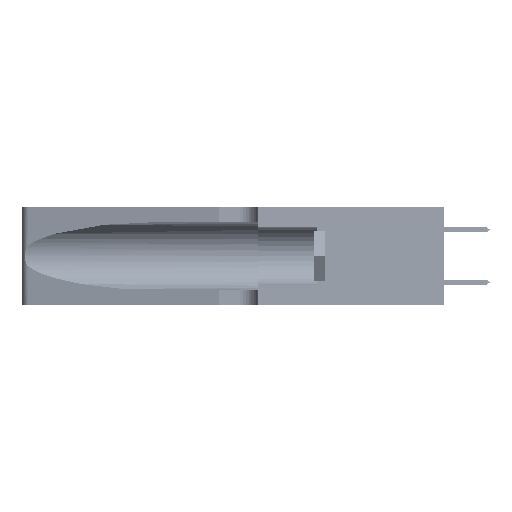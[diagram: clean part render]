
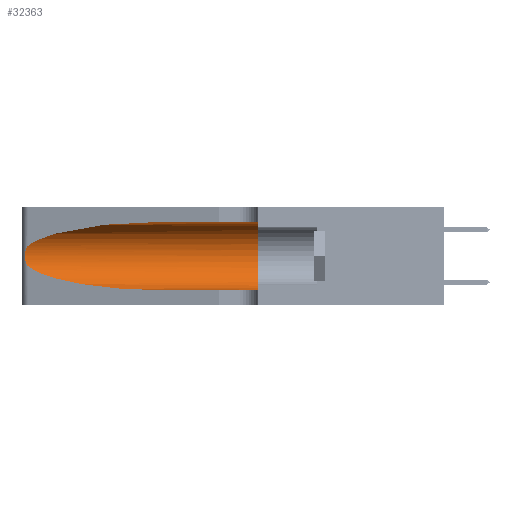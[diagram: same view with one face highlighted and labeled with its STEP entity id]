
A CAD part, left-side view. The second image highlights one B-rep face of the part: STEP entity #32363.
In plain terms, the highlighted cylindrical face has radius 3.308 mm (diameter 6.617 mm), a partial arc.
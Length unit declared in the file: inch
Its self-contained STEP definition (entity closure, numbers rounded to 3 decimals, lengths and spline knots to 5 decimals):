
#355 = CARTESIAN_POINT ( 'NONE',  ( 0.2373, 1.15595, 0.28018 ) ) ;
#601 = VERTEX_POINT ( 'NONE', #27630 ) ;
#756 = VERTEX_POINT ( 'NONE', #24742 ) ;
#3190 = DIRECTION ( 'NONE',  ( 0., 0., 1. ) ) ;
#3451 = CARTESIAN_POINT ( 'NONE',  ( 0.26075, 1.23896, 0.178 ) ) ;
#3780 = CARTESIAN_POINT ( 'NONE',  ( 0.25555, 1.22994, 0.2215 ) ) ;
#4079 = DIRECTION ( 'NONE',  ( 0., -1., 0. ) ) ;
#5245 = AXIS2_PLACEMENT_3D ( 'NONE', #41445, #26483, #3190 ) ;
#6985 = EDGE_CURVE ( 'NONE', #756, #44145, #25045, .T. ) ;
#7262 =( BOUNDED_CURVE ( )  B_SPLINE_CURVE ( 3, ( #23469, #15491, #355, #7610 ),
 .UNSPECIFIED., .F., .T. ) 
 B_SPLINE_CURVE_WITH_KNOTS ( ( 4, 4 ),
 ( 1.5708, 2.84003 ),
 .UNSPECIFIED. ) 
 CURVE ( )  GEOMETRIC_REPRESENTATION_ITEM ( )  RATIONAL_B_SPLINE_CURVE ( ( 1., 0.87, 0.87, 1. ) ) 
 REPRESENTATION_ITEM ( '' )  );
#7610 = CARTESIAN_POINT ( 'NONE',  ( 0.25487, 1.22718, 0.22369 ) ) ;
#7675 = CARTESIAN_POINT ( 'NONE',  ( 0.18966, 0.96281, 0.05475 ) ) ;
#11560 = CARTESIAN_POINT ( 'NONE',  ( 0.1305, 0.72297, 0.05475 ) ) ;
#13143 = DIRECTION ( 'NONE',  ( 0., 0., -1. ) ) ;
#13165 = VECTOR ( 'NONE', #28298, 39.37008 ) ;
#14161 = CARTESIAN_POINT ( 'NONE',  ( 0.1305, 1.61858, 0.05475 ) ) ;
#14622 = EDGE_LOOP ( 'NONE', ( #31827, #27437, #39032, #21036, #49665, #19618 ) ) ;
#14868 = CARTESIAN_POINT ( 'NONE',  ( 0.25639, 1.23184, 0.21858 ) ) ;
#15491 = CARTESIAN_POINT ( 'NONE',  ( 0.18966, 0.96281, 0.31525 ) ) ;
#15770 = VERTEX_POINT ( 'NONE', #45785 ) ;
#15894 = CARTESIAN_POINT ( 'NONE',  ( 0.25487, 1.22718, 0.14631 ) ) ;
#18370 = CARTESIAN_POINT ( 'NONE',  ( 0.26017, 1.23833, 0.17102 ) ) ;
#18855 = CARTESIAN_POINT ( 'NONE',  ( 0.25487, 1.22718, 0.22369 ) ) ;
#19618 = ORIENTED_EDGE ( 'NONE', *, *, #22628, .F. ) ;
#19921 = VERTEX_POINT ( 'NONE', #23820 ) ;
#21036 = ORIENTED_EDGE ( 'NONE', *, *, #43276, .T. ) ;
#22287 = EDGE_CURVE ( 'NONE', #15770, #601, #47405, .T. ) ;
#22376 = CARTESIAN_POINT ( 'NONE',  ( 0.25856, 1.23593, 0.16098 ) ) ;
#22574 = CARTESIAN_POINT ( 'NONE',  ( 0.1305, 0.72297, 0.31525 ) ) ;
#22628 = EDGE_CURVE ( 'NONE', #37428, #15770, #25726, .T. ) ;
#22677 = DIRECTION ( 'NONE',  ( 0., -1., 0. ) ) ;
#23313 = LINE ( 'NONE', #14161, #41933 ) ;
#23469 = CARTESIAN_POINT ( 'NONE',  ( 0.1305, 0.72297, 0.31525 ) ) ;
#23820 = CARTESIAN_POINT ( 'NONE',  ( 0.1305, 0.72297, 0.05475 ) ) ;
#24742 = CARTESIAN_POINT ( 'NONE',  ( 0.25487, 1.22718, 0.22369 ) ) ;
#25032 = FACE_OUTER_BOUND ( 'NONE', #14622, .T. ) ;
#25045 = B_SPLINE_CURVE_WITH_KNOTS ( 'NONE', 3,
 ( #18855, #3780, #14868, #41863, #45380, #49560, #38152, #3451, #18370, #22376, #30262, #31138, #26567, #41529 ),
 .UNSPECIFIED., .F., .F.,
 ( 4, 2, 2, 2, 2, 2, 4 ),
 ( 0., 0.00027, 0.00053, 0.00107, 0.0016, 0.00187, 0.00214 ),
 .UNSPECIFIED. ) ;
#25278 = EDGE_CURVE ( 'NONE', #37428, #756, #7262, .T. ) ;
#25726 = LINE ( 'NONE', #43092, #13165 ) ;
#26483 = DIRECTION ( 'NONE',  ( 0., 1., 0. ) ) ;
#26567 = CARTESIAN_POINT ( 'NONE',  ( 0.25555, 1.22993, 0.14849 ) ) ;
#27437 = ORIENTED_EDGE ( 'NONE', *, *, #6985, .T. ) ;
#27630 = CARTESIAN_POINT ( 'NONE',  ( 0.1305, 0.35, 0.05475 ) ) ;
#28298 = DIRECTION ( 'NONE',  ( 0., -1., 0. ) ) ;
#30262 = CARTESIAN_POINT ( 'NONE',  ( 0.25789, 1.23486, 0.15765 ) ) ;
#30290 =( BOUNDED_CURVE ( )  B_SPLINE_CURVE ( 3, ( #38504, #34673, #7675, #11560 ),
 .UNSPECIFIED., .F., .T. ) 
 B_SPLINE_CURVE_WITH_KNOTS ( ( 4, 4 ),
 ( 3.44316, 4.71239 ),
 .UNSPECIFIED. ) 
 CURVE ( )  GEOMETRIC_REPRESENTATION_ITEM ( )  RATIONAL_B_SPLINE_CURVE ( ( 1., 0.87, 0.87, 1. ) ) 
 REPRESENTATION_ITEM ( '' )  );
#31138 = CARTESIAN_POINT ( 'NONE',  ( 0.25639, 1.23186, 0.15144 ) ) ;
#31502 = EDGE_CURVE ( 'NONE', #44145, #19921, #30290, .T. ) ;
#31827 = ORIENTED_EDGE ( 'NONE', *, *, #25278, .T. ) ;
#32363 = ADVANCED_FACE ( 'NONE', ( #25032 ), #34714, .F. ) ;
#34673 = CARTESIAN_POINT ( 'NONE',  ( 0.2373, 1.15595, 0.08982 ) ) ;
#34714 = CYLINDRICAL_SURFACE ( 'NONE', #42370, 0.13025 ) ;
#34934 = CARTESIAN_POINT ( 'NONE',  ( 0.1305, 1.61858, 0.185 ) ) ;
#37428 = VERTEX_POINT ( 'NONE', #22574 ) ;
#38152 = CARTESIAN_POINT ( 'NONE',  ( 0.26075, 1.23896, 0.19203 ) ) ;
#38504 = CARTESIAN_POINT ( 'NONE',  ( 0.25487, 1.22718, 0.14631 ) ) ;
#39032 = ORIENTED_EDGE ( 'NONE', *, *, #31502, .T. ) ;
#41445 = CARTESIAN_POINT ( 'NONE',  ( 0.1305, 0.35, 0.185 ) ) ;
#41529 = CARTESIAN_POINT ( 'NONE',  ( 0.25487, 1.22718, 0.14631 ) ) ;
#41863 = CARTESIAN_POINT ( 'NONE',  ( 0.25787, 1.23484, 0.2124 ) ) ;
#41933 = VECTOR ( 'NONE', #22677, 39.37008 ) ;
#42370 = AXIS2_PLACEMENT_3D ( 'NONE', #34934, #4079, #13143 ) ;
#43092 = CARTESIAN_POINT ( 'NONE',  ( 0.1305, 1.61858, 0.31525 ) ) ;
#43276 = EDGE_CURVE ( 'NONE', #19921, #601, #23313, .T. ) ;
#44145 = VERTEX_POINT ( 'NONE', #15894 ) ;
#45380 = CARTESIAN_POINT ( 'NONE',  ( 0.25854, 1.2359, 0.20912 ) ) ;
#45785 = CARTESIAN_POINT ( 'NONE',  ( 0.1305, 0.35, 0.31525 ) ) ;
#47405 = CIRCLE ( 'NONE', #5245, 0.13025 ) ;
#49560 = CARTESIAN_POINT ( 'NONE',  ( 0.26018, 1.23835, 0.19895 ) ) ;
#49665 = ORIENTED_EDGE ( 'NONE', *, *, #22287, .F. ) ;
